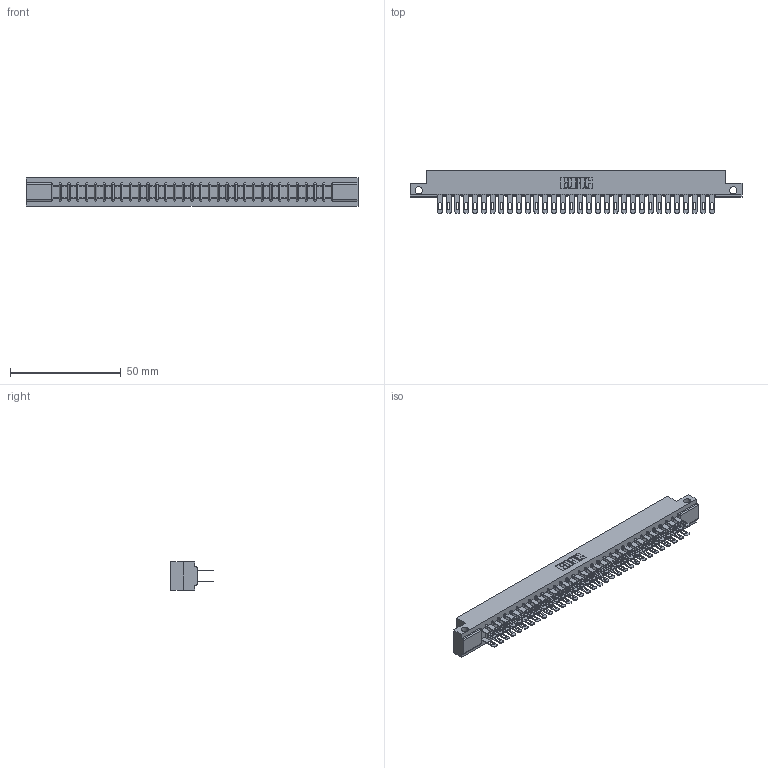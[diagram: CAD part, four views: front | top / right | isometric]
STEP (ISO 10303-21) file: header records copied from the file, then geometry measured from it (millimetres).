
FILE_DESCRIPTION (( 'STEP AP203' ), '1' );
FILE_NAME ('357-064-400-212.STEP', '2020-10-04T16:19:05', ( '' ), ( '' ), 'SwSTEP 2.0', 'SolidWorks 2020', '' );
FILE_SCHEMA (( 'CONFIG_CONTROL_DESIGN' ));
Length unit declared in the file: inch
Products named in the file (3): 307 Part_.128 Dia Side Mounting Holes; 357-064-400-212; 307-290-001_500
Assembly tree (65 placements, depth 2):
  357-064-400-212
    307 Part_.128 Dia Side Mounting Holes
    307-290-001_500  x64
Bounding box: 149.81 x 19.18 x 12.7 mm (x, y, z)
Volume: 15900.8 mm3; surface area: 20257.8 mm2
Topology: 65 solids, 65 shells, 3095 faces, 8643 edges, 5586 vertices
Faces by surface type: plane 1990, cylinder 1039, sphere 66
Entity records: 29666 total; most frequent: CARTESIAN_POINT 4852, ORIENTED_EDGE 4806, DIRECTION 4759, EDGE_CURVE 2403, LINE 1837, VECTOR 1837, VERTEX_POINT 1554, AXIS2_PLACEMENT_3D 1461
